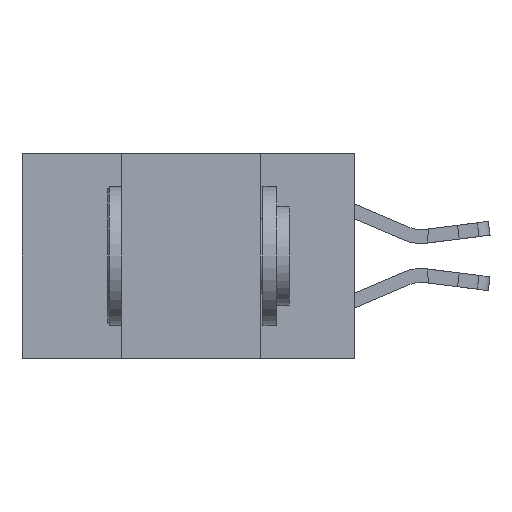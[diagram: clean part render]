
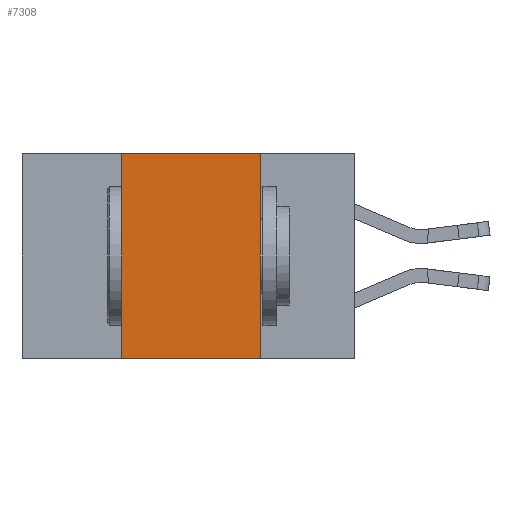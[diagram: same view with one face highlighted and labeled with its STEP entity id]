
A CAD part, left-side view. The second image highlights one B-rep face of the part: STEP entity #7308.
In plain terms, the highlighted planar face has unit normal (-1, 0, 0).
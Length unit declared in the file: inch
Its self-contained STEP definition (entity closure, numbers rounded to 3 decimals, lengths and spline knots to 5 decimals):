
#297 = DIRECTION ( 'NONE',  ( 1., 0., 0. ) ) ;
#988 = ORIENTED_EDGE ( 'NONE', *, *, #5984, .F. ) ;
#1938 = LINE ( 'NONE', #7723, #15052 ) ;
#2926 = DIRECTION ( 'NONE',  ( 0., -1., 0. ) ) ;
#3413 = VERTEX_POINT ( 'NONE', #8782 ) ;
#3973 = DIRECTION ( 'NONE',  ( 0., 0., -1. ) ) ;
#3995 = AXIS2_PLACEMENT_3D ( 'NONE', #10125, #297, #11802 ) ;
#4150 = VERTEX_POINT ( 'NONE', #7625 ) ;
#4283 = EDGE_LOOP ( 'NONE', ( #13100, #17283, #988, #5370 ) ) ;
#4844 = EDGE_CURVE ( 'NONE', #4150, #9146, #1938, .T. ) ;
#5370 = ORIENTED_EDGE ( 'NONE', *, *, #4844, .T. ) ;
#5880 = LINE ( 'NONE', #11188, #14103 ) ;
#5984 = EDGE_CURVE ( 'NONE', #4150, #18689, #10937, .T. ) ;
#6577 = VECTOR ( 'NONE', #19378, 39.37008 ) ;
#6620 = CARTESIAN_POINT ( 'NONE',  ( 0., 0.42, 0. ) ) ;
#7308 = ADVANCED_FACE ( 'NONE', ( #18978 ), #18122, .F. ) ;
#7625 = CARTESIAN_POINT ( 'NONE',  ( 0., 0.42, -0.37 ) ) ;
#7723 = CARTESIAN_POINT ( 'NONE',  ( 0., 0.6, -0.37 ) ) ;
#8166 = EDGE_CURVE ( 'NONE', #3413, #9146, #17284, .T. ) ;
#8456 = EDGE_CURVE ( 'NONE', #18689, #3413, #5880, .T. ) ;
#8782 = CARTESIAN_POINT ( 'NONE',  ( 0., 0.17, 0. ) ) ;
#8877 = CARTESIAN_POINT ( 'NONE',  ( 0., 0.17, 0. ) ) ;
#9146 = VERTEX_POINT ( 'NONE', #16319 ) ;
#10125 = CARTESIAN_POINT ( 'NONE',  ( 0., 0.6, 0. ) ) ;
#10937 = LINE ( 'NONE', #6620, #6577 ) ;
#11188 = CARTESIAN_POINT ( 'NONE',  ( 0., 0.6, 0. ) ) ;
#11341 = VECTOR ( 'NONE', #3973, 39.37008 ) ;
#11802 = DIRECTION ( 'NONE',  ( 0., 0., -1. ) ) ;
#13100 = ORIENTED_EDGE ( 'NONE', *, *, #8166, .F. ) ;
#13239 = CARTESIAN_POINT ( 'NONE',  ( 0., 0.42, 0. ) ) ;
#14103 = VECTOR ( 'NONE', #2926, 39.37008 ) ;
#15052 = VECTOR ( 'NONE', #16203, 39.37008 ) ;
#16203 = DIRECTION ( 'NONE',  ( 0., -1., 0. ) ) ;
#16319 = CARTESIAN_POINT ( 'NONE',  ( 0., 0.17, -0.37 ) ) ;
#17283 = ORIENTED_EDGE ( 'NONE', *, *, #8456, .F. ) ;
#17284 = LINE ( 'NONE', #8877, #11341 ) ;
#18122 = PLANE ( 'NONE',  #3995 ) ;
#18689 = VERTEX_POINT ( 'NONE', #13239 ) ;
#18978 = FACE_OUTER_BOUND ( 'NONE', #4283, .T. ) ;
#19378 = DIRECTION ( 'NONE',  ( 0., 0., 1. ) ) ;
